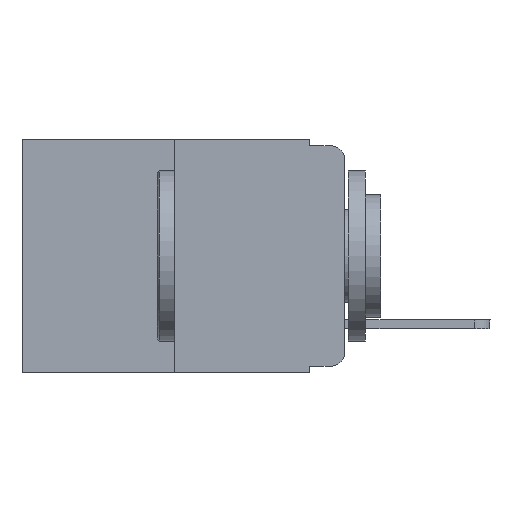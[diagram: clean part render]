
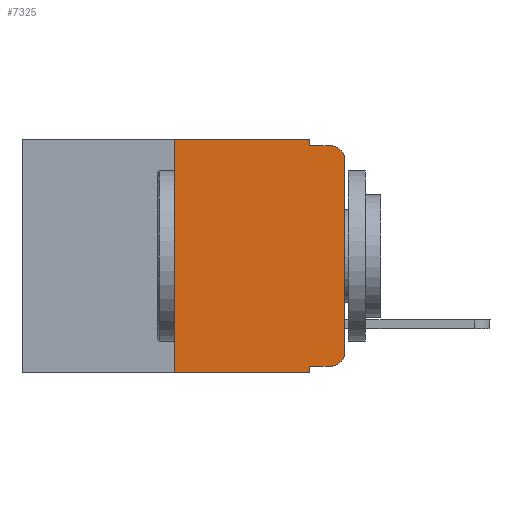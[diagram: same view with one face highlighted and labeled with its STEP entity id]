
A CAD part, left-side view. The second image highlights one B-rep face of the part: STEP entity #7325.
In plain terms, the highlighted planar face has unit normal (-1, 0, 0).
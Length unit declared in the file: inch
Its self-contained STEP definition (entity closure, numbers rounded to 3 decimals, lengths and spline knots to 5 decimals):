
#117 = CARTESIAN_POINT ( 'NONE',  ( 0., 0.051, 0. ) ) ;
#199 = DIRECTION ( 'NONE',  ( 0., -1., 0. ) ) ;
#560 = VECTOR ( 'NONE', #18382, 39.37008 ) ;
#855 = DIRECTION ( 'NONE',  ( 0., 0., -1. ) ) ;
#970 = VERTEX_POINT ( 'NONE', #9687 ) ;
#1602 = LINE ( 'NONE', #7966, #17181 ) ;
#1702 = ORIENTED_EDGE ( 'NONE', *, *, #4744, .T. ) ;
#1874 = CARTESIAN_POINT ( 'NONE',  ( 0., 0., -0.03 ) ) ;
#1947 = ORIENTED_EDGE ( 'NONE', *, *, #19117, .F. ) ;
#2459 = DIRECTION ( 'NONE',  ( -1., 0., 0. ) ) ;
#2780 = CARTESIAN_POINT ( 'NONE',  ( 0., 0.473, -0.343 ) ) ;
#2962 = CARTESIAN_POINT ( 'NONE',  ( 0., 0., 0. ) ) ;
#3031 = CARTESIAN_POINT ( 'NONE',  ( 0., 0.25, 0. ) ) ;
#3094 = ORIENTED_EDGE ( 'NONE', *, *, #18822, .T. ) ;
#3394 = VECTOR ( 'NONE', #9523, 39.37008 ) ;
#3412 = CARTESIAN_POINT ( 'NONE',  ( 0., 0.051, 0. ) ) ;
#3620 = VERTEX_POINT ( 'NONE', #3412 ) ;
#3801 = EDGE_LOOP ( 'NONE', ( #1702, #3094, #1947, #12487, #15481, #10622, #12666, #10441, #20029, #9383 ) ) ;
#4744 = EDGE_CURVE ( 'NONE', #7368, #15224, #6921, .T. ) ;
#6104 = DIRECTION ( 'NONE',  ( 0., 0., -1. ) ) ;
#6126 = CARTESIAN_POINT ( 'NONE',  ( 0., 0.02, -0.01 ) ) ;
#6489 = CARTESIAN_POINT ( 'NONE',  ( 0., 0.051, -0.333 ) ) ;
#6781 = VERTEX_POINT ( 'NONE', #7537 ) ;
#6870 = DIRECTION ( 'NONE',  ( -1., 0., 0. ) ) ;
#6921 = LINE ( 'NONE', #2962, #560 ) ;
#7325 = ADVANCED_FACE ( 'NONE', ( #18951 ), #18572, .F. ) ;
#7368 = VERTEX_POINT ( 'NONE', #13968 ) ;
#7532 = EDGE_CURVE ( 'NONE', #3620, #970, #19202, .T. ) ;
#7537 = CARTESIAN_POINT ( 'NONE',  ( 0., 0.051, -0.343 ) ) ;
#7746 = CARTESIAN_POINT ( 'NONE',  ( 0., 0.051, -0.01 ) ) ;
#7966 = CARTESIAN_POINT ( 'NONE',  ( 0., 0.473, 0. ) ) ;
#8677 = LINE ( 'NONE', #13559, #8906 ) ;
#8870 = EDGE_CURVE ( 'NONE', #17365, #7368, #11193, .T. ) ;
#8906 = VECTOR ( 'NONE', #16551, 39.37008 ) ;
#9008 = VECTOR ( 'NONE', #14177, 39.37008 ) ;
#9184 = AXIS2_PLACEMENT_3D ( 'NONE', #10141, #6870, #17867 ) ;
#9383 = ORIENTED_EDGE ( 'NONE', *, *, #8870, .T. ) ;
#9466 = AXIS2_PLACEMENT_3D ( 'NONE', #19577, #2459, #855 ) ;
#9506 = CIRCLE ( 'NONE', #9184, 0.02 ) ;
#9523 = DIRECTION ( 'NONE',  ( 0., -1., 0. ) ) ;
#9687 = CARTESIAN_POINT ( 'NONE',  ( 0., 0.051, -0.01 ) ) ;
#9743 = LINE ( 'NONE', #7746, #3394 ) ;
#9803 = CARTESIAN_POINT ( 'NONE',  ( 0., 0.25, 0. ) ) ;
#10104 = CARTESIAN_POINT ( 'NONE',  ( 0., 0.051, -0.333 ) ) ;
#10117 = VECTOR ( 'NONE', #15490, 39.37008 ) ;
#10141 = CARTESIAN_POINT ( 'NONE',  ( 0., 0.02, -0.03 ) ) ;
#10441 = ORIENTED_EDGE ( 'NONE', *, *, #14543, .F. ) ;
#10519 = EDGE_CURVE ( 'NONE', #15644, #3620, #1602, .T. ) ;
#10622 = ORIENTED_EDGE ( 'NONE', *, *, #11823, .F. ) ;
#10815 = VERTEX_POINT ( 'NONE', #10104 ) ;
#11155 = EDGE_CURVE ( 'NONE', #10815, #17365, #16948, .T. ) ;
#11193 = CIRCLE ( 'NONE', #9466, 0.02 ) ;
#11503 = DIRECTION ( 'NONE',  ( 0., 0., 1. ) ) ;
#11823 = EDGE_CURVE ( 'NONE', #17044, #15644, #16685, .T. ) ;
#12131 = DIRECTION ( 'NONE',  ( 1., 0., 0. ) ) ;
#12210 = CARTESIAN_POINT ( 'NONE',  ( 0., 0.473, 0. ) ) ;
#12487 = ORIENTED_EDGE ( 'NONE', *, *, #7532, .F. ) ;
#12666 = ORIENTED_EDGE ( 'NONE', *, *, #13093, .T. ) ;
#13093 = EDGE_CURVE ( 'NONE', #17044, #6781, #17620, .T. ) ;
#13559 = CARTESIAN_POINT ( 'NONE',  ( 0., 0.051, 0. ) ) ;
#13968 = CARTESIAN_POINT ( 'NONE',  ( 0., 0., -0.313 ) ) ;
#13988 = CARTESIAN_POINT ( 'NONE',  ( 0., 0.02, -0.333 ) ) ;
#14177 = DIRECTION ( 'NONE',  ( 0., 0., -1. ) ) ;
#14543 = EDGE_CURVE ( 'NONE', #10815, #6781, #8677, .T. ) ;
#15008 = CARTESIAN_POINT ( 'NONE',  ( 0., 0.25, -0.343 ) ) ;
#15224 = VERTEX_POINT ( 'NONE', #1874 ) ;
#15475 = VECTOR ( 'NONE', #11503, 39.37008 ) ;
#15481 = ORIENTED_EDGE ( 'NONE', *, *, #10519, .F. ) ;
#15490 = DIRECTION ( 'NONE',  ( 0., -1., 0. ) ) ;
#15644 = VERTEX_POINT ( 'NONE', #3031 ) ;
#15821 = DIRECTION ( 'NONE',  ( 0., -1., 0. ) ) ;
#16551 = DIRECTION ( 'NONE',  ( 0., 0., -1. ) ) ;
#16685 = LINE ( 'NONE', #9803, #15475 ) ;
#16948 = LINE ( 'NONE', #6489, #19863 ) ;
#17044 = VERTEX_POINT ( 'NONE', #15008 ) ;
#17181 = VECTOR ( 'NONE', #15821, 39.37008 ) ;
#17227 = VERTEX_POINT ( 'NONE', #6126 ) ;
#17365 = VERTEX_POINT ( 'NONE', #13988 ) ;
#17620 = LINE ( 'NONE', #2780, #10117 ) ;
#17867 = DIRECTION ( 'NONE',  ( 0., 0., -1. ) ) ;
#18382 = DIRECTION ( 'NONE',  ( 0., 0., 1. ) ) ;
#18572 = PLANE ( 'NONE',  #20083 ) ;
#18822 = EDGE_CURVE ( 'NONE', #15224, #17227, #9506, .T. ) ;
#18951 = FACE_OUTER_BOUND ( 'NONE', #3801, .T. ) ;
#19117 = EDGE_CURVE ( 'NONE', #970, #17227, #9743, .T. ) ;
#19202 = LINE ( 'NONE', #117, #9008 ) ;
#19577 = CARTESIAN_POINT ( 'NONE',  ( 0., 0.02, -0.313 ) ) ;
#19863 = VECTOR ( 'NONE', #199, 39.37008 ) ;
#20029 = ORIENTED_EDGE ( 'NONE', *, *, #11155, .T. ) ;
#20083 = AXIS2_PLACEMENT_3D ( 'NONE', #12210, #12131, #6104 ) ;
